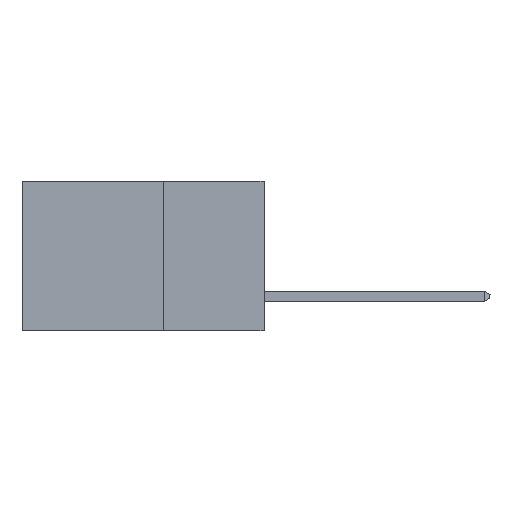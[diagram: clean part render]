
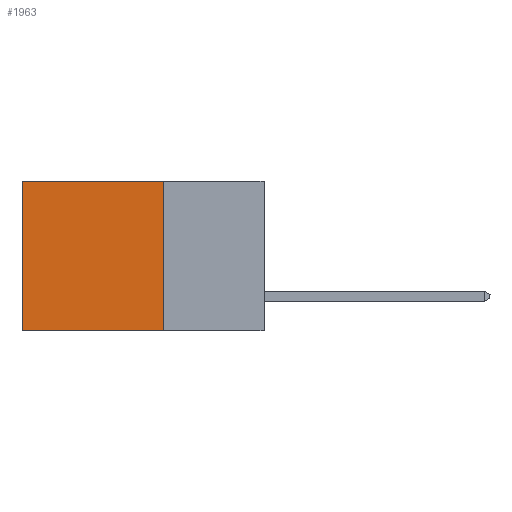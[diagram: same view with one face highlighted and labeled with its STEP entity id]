
A CAD part, left-side view. The second image highlights one B-rep face of the part: STEP entity #1963.
In plain terms, the highlighted planar face has unit normal (-1, 0, 0).
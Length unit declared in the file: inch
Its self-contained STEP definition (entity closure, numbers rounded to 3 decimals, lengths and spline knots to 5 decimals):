
#50 = CARTESIAN_POINT ( 'NONE',  ( 0.2615, 0.6, -0.37 ) ) ;
#325 = CARTESIAN_POINT ( 'NONE',  ( 0.2615, 0.25, 0. ) ) ;
#443 = CARTESIAN_POINT ( 'NONE',  ( 0.2615, 0.6, -0.37 ) ) ;
#447 = ORIENTED_EDGE ( 'NONE', *, *, #4466, .T. ) ;
#773 = DIRECTION ( 'NONE',  ( 0., 0., -1. ) ) ;
#990 = CARTESIAN_POINT ( 'NONE',  ( 0.2615, 0.25, -0.37 ) ) ;
#1297 = ORIENTED_EDGE ( 'NONE', *, *, #7595, .T. ) ;
#1519 = VECTOR ( 'NONE', #773, 39.37008 ) ;
#1963 = ADVANCED_FACE ( 'NONE', ( #5462 ), #9141, .F. ) ;
#1977 = DIRECTION ( 'NONE',  ( 0., 0., -1. ) ) ;
#2255 = ORIENTED_EDGE ( 'NONE', *, *, #3070, .F. ) ;
#3070 = EDGE_CURVE ( 'NONE', #7187, #10001, #10441, .T. ) ;
#3223 = CARTESIAN_POINT ( 'NONE',  ( 0.2615, 0.25, 0. ) ) ;
#3290 = ORIENTED_EDGE ( 'NONE', *, *, #5293, .F. ) ;
#4096 = DIRECTION ( 'NONE',  ( 0., 1., 0. ) ) ;
#4466 = EDGE_CURVE ( 'NONE', #7187, #9151, #5595, .T. ) ;
#4783 = DIRECTION ( 'NONE',  ( 1., 0., 0. ) ) ;
#5175 = LINE ( 'NONE', #443, #1519 ) ;
#5293 = EDGE_CURVE ( 'NONE', #10001, #7314, #10860, .T. ) ;
#5462 = FACE_OUTER_BOUND ( 'NONE', #7969, .T. ) ;
#5536 = VECTOR ( 'NONE', #4096, 39.37008 ) ;
#5595 = LINE ( 'NONE', #325, #5536 ) ;
#5694 = VECTOR ( 'NONE', #6444, 39.37008 ) ;
#6020 = CARTESIAN_POINT ( 'NONE',  ( 0.2615, 0.25, -0.37 ) ) ;
#6444 = DIRECTION ( 'NONE',  ( 0., 1., 0. ) ) ;
#7187 = VERTEX_POINT ( 'NONE', #3223 ) ;
#7314 = VERTEX_POINT ( 'NONE', #50 ) ;
#7595 = EDGE_CURVE ( 'NONE', #9151, #7314, #5175, .T. ) ;
#7650 = CARTESIAN_POINT ( 'NONE',  ( 0.2615, 0.25, -0.37 ) ) ;
#7969 = EDGE_LOOP ( 'NONE', ( #1297, #3290, #2255, #447 ) ) ;
#8288 = VECTOR ( 'NONE', #9581, 39.37008 ) ;
#8998 = AXIS2_PLACEMENT_3D ( 'NONE', #9904, #4783, #1977 ) ;
#9141 = PLANE ( 'NONE',  #8998 ) ;
#9151 = VERTEX_POINT ( 'NONE', #11002 ) ;
#9581 = DIRECTION ( 'NONE',  ( 0., 0., -1. ) ) ;
#9904 = CARTESIAN_POINT ( 'NONE',  ( 0.2615, 0.25, -0.37 ) ) ;
#10001 = VERTEX_POINT ( 'NONE', #7650 ) ;
#10441 = LINE ( 'NONE', #6020, #8288 ) ;
#10860 = LINE ( 'NONE', #990, #5694 ) ;
#11002 = CARTESIAN_POINT ( 'NONE',  ( 0.2615, 0.6, 0. ) ) ;
